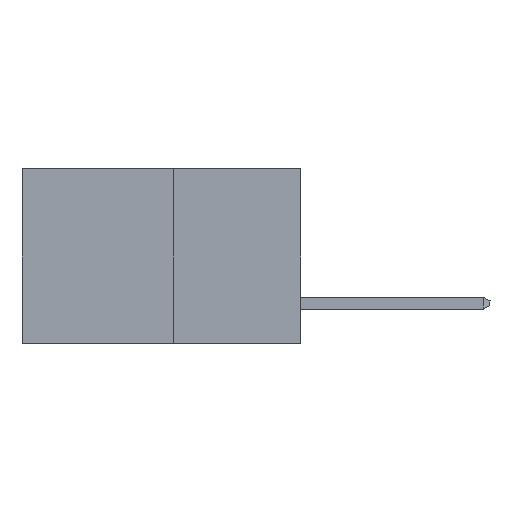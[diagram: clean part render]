
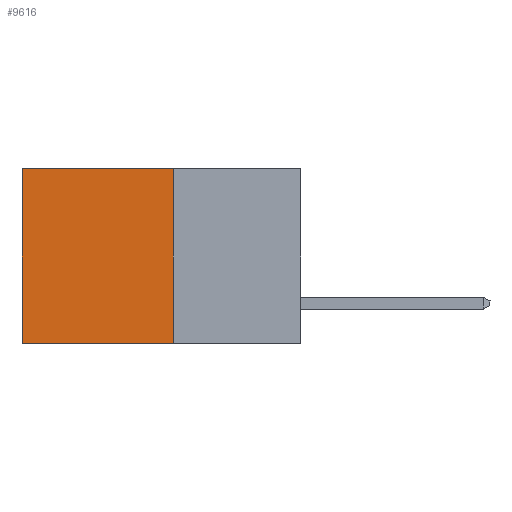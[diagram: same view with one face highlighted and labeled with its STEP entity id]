
A CAD part, left-side view. The second image highlights one B-rep face of the part: STEP entity #9616.
In plain terms, the highlighted planar face has unit normal (-1, 0, 0).
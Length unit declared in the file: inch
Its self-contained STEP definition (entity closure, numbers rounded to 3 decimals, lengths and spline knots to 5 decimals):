
#309 = LINE ( 'NONE', #1011, #24862 ) ;
#1011 = CARTESIAN_POINT ( 'NONE',  ( 0.277, 0.27, 0. ) ) ;
#3703 = ORIENTED_EDGE ( 'NONE', *, *, #15279, .F. ) ;
#4145 = CARTESIAN_POINT ( 'NONE',  ( 0.277, 0.27, -0.37 ) ) ;
#4504 = DIRECTION ( 'NONE',  ( 0., 0., -1. ) ) ;
#4536 = DIRECTION ( 'NONE',  ( 1., 0., 0. ) ) ;
#4602 = CARTESIAN_POINT ( 'NONE',  ( 0.277, 0.27, -0.37 ) ) ;
#4641 = PLANE ( 'NONE',  #11885 ) ;
#4860 = CARTESIAN_POINT ( 'NONE',  ( 0.277, 0.27, 0. ) ) ;
#6351 = CARTESIAN_POINT ( 'NONE',  ( 0.277, 0.27, -0.37 ) ) ;
#6545 = DIRECTION ( 'NONE',  ( 0., 1., 0. ) ) ;
#7029 = LINE ( 'NONE', #6351, #19006 ) ;
#8404 = LINE ( 'NONE', #26512, #19637 ) ;
#9616 = ADVANCED_FACE ( 'NONE', ( #26342 ), #4641, .F. ) ;
#10402 = EDGE_CURVE ( 'NONE', #10672, #12688, #7029, .T. ) ;
#10672 = VERTEX_POINT ( 'NONE', #4860 ) ;
#11885 = AXIS2_PLACEMENT_3D ( 'NONE', #4602, #4536, #4504 ) ;
#12688 = VERTEX_POINT ( 'NONE', #21874 ) ;
#13530 = ORIENTED_EDGE ( 'NONE', *, *, #27143, .T. ) ;
#14791 = DIRECTION ( 'NONE',  ( 0., 0., -1. ) ) ;
#15110 = VERTEX_POINT ( 'NONE', #24917 ) ;
#15279 = EDGE_CURVE ( 'NONE', #12688, #18891, #16884, .T. ) ;
#16884 = LINE ( 'NONE', #4145, #28507 ) ;
#18891 = VERTEX_POINT ( 'NONE', #28848 ) ;
#19006 = VECTOR ( 'NONE', #25309, 39.37008 ) ;
#19637 = VECTOR ( 'NONE', #14791, 39.37008 ) ;
#20112 = DIRECTION ( 'NONE',  ( 0., 1., 0. ) ) ;
#21874 = CARTESIAN_POINT ( 'NONE',  ( 0.277, 0.27, -0.37 ) ) ;
#24862 = VECTOR ( 'NONE', #20112, 39.37008 ) ;
#24917 = CARTESIAN_POINT ( 'NONE',  ( 0.277, 0.59, 0. ) ) ;
#25309 = DIRECTION ( 'NONE',  ( 0., 0., -1. ) ) ;
#26342 = FACE_OUTER_BOUND ( 'NONE', #29541, .T. ) ;
#26512 = CARTESIAN_POINT ( 'NONE',  ( 0.277, 0.59, -0.37 ) ) ;
#27143 = EDGE_CURVE ( 'NONE', #10672, #15110, #309, .T. ) ;
#27627 = ORIENTED_EDGE ( 'NONE', *, *, #10402, .F. ) ;
#28507 = VECTOR ( 'NONE', #6545, 39.37008 ) ;
#28848 = CARTESIAN_POINT ( 'NONE',  ( 0.277, 0.59, -0.37 ) ) ;
#28878 = ORIENTED_EDGE ( 'NONE', *, *, #29135, .T. ) ;
#29135 = EDGE_CURVE ( 'NONE', #15110, #18891, #8404, .T. ) ;
#29541 = EDGE_LOOP ( 'NONE', ( #28878, #3703, #27627, #13530 ) ) ;
